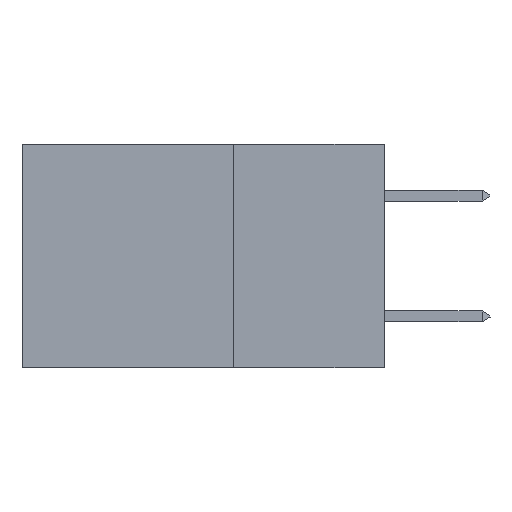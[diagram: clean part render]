
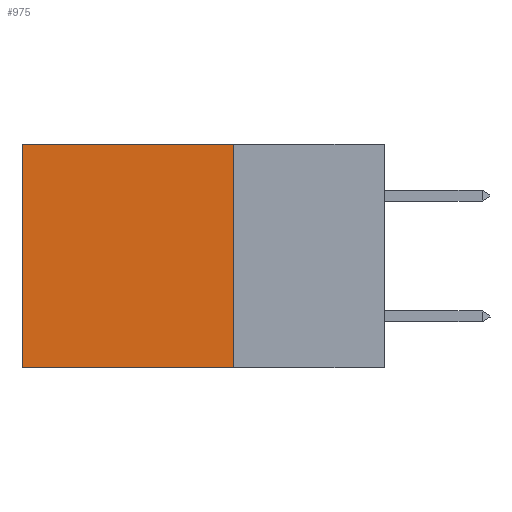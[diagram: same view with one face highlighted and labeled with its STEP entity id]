
A CAD part, left-side view. The second image highlights one B-rep face of the part: STEP entity #975.
In plain terms, the highlighted planar face has unit normal (-1, 0, 0).
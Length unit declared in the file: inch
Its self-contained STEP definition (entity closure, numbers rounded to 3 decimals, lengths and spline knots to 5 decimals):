
#78 = CARTESIAN_POINT ( 'NONE',  ( 0.2875, 0.25, 0. ) ) ;
#312 = DIRECTION ( 'NONE',  ( 0., 1., 0. ) ) ;
#412 = ORIENTED_EDGE ( 'NONE', *, *, #5667, .T. ) ;
#666 = ORIENTED_EDGE ( 'NONE', *, *, #23189, .F. ) ;
#975 = ADVANCED_FACE ( 'NONE', ( #8266 ), #23697, .F. ) ;
#1405 = CARTESIAN_POINT ( 'NONE',  ( 0.2875, 0.25, -0.37 ) ) ;
#1751 = DIRECTION ( 'NONE',  ( 0., 0., -1. ) ) ;
#2479 = CARTESIAN_POINT ( 'NONE',  ( 0.2875, 0.25, 0. ) ) ;
#2648 = LINE ( 'NONE', #6725, #13887 ) ;
#2697 = ORIENTED_EDGE ( 'NONE', *, *, #15838, .T. ) ;
#2740 = DIRECTION ( 'NONE',  ( 0., 0., -1. ) ) ;
#2899 = DIRECTION ( 'NONE',  ( 1., 0., 0. ) ) ;
#3260 = AXIS2_PLACEMENT_3D ( 'NONE', #23617, #2899, #2740 ) ;
#3999 = VECTOR ( 'NONE', #13714, 39.37008 ) ;
#4315 = LINE ( 'NONE', #2479, #3999 ) ;
#5667 = EDGE_CURVE ( 'NONE', #8730, #23796, #6262, .T. ) ;
#6262 = LINE ( 'NONE', #7137, #14560 ) ;
#6541 = CARTESIAN_POINT ( 'NONE',  ( 0.2875, 0.6, -0.37 ) ) ;
#6725 = CARTESIAN_POINT ( 'NONE',  ( 0.2875, 0.25, -0.37 ) ) ;
#7029 = CARTESIAN_POINT ( 'NONE',  ( 0.2875, 0.6, 0. ) ) ;
#7137 = CARTESIAN_POINT ( 'NONE',  ( 0.2875, 0.25, 0. ) ) ;
#8266 = FACE_OUTER_BOUND ( 'NONE', #23594, .T. ) ;
#8289 = CARTESIAN_POINT ( 'NONE',  ( 0.2875, 0.6, 0. ) ) ;
#8730 = VERTEX_POINT ( 'NONE', #78 ) ;
#9624 = EDGE_CURVE ( 'NONE', #11899, #20979, #2648, .T. ) ;
#11899 = VERTEX_POINT ( 'NONE', #1405 ) ;
#13714 = DIRECTION ( 'NONE',  ( 0., 0., -1. ) ) ;
#13887 = VECTOR ( 'NONE', #24391, 39.37008 ) ;
#14025 = LINE ( 'NONE', #7029, #23898 ) ;
#14560 = VECTOR ( 'NONE', #312, 39.37008 ) ;
#15838 = EDGE_CURVE ( 'NONE', #23796, #20979, #14025, .T. ) ;
#16441 = ORIENTED_EDGE ( 'NONE', *, *, #9624, .F. ) ;
#20979 = VERTEX_POINT ( 'NONE', #6541 ) ;
#23189 = EDGE_CURVE ( 'NONE', #8730, #11899, #4315, .T. ) ;
#23594 = EDGE_LOOP ( 'NONE', ( #2697, #16441, #666, #412 ) ) ;
#23617 = CARTESIAN_POINT ( 'NONE',  ( 0.2875, 0.25, 0. ) ) ;
#23697 = PLANE ( 'NONE',  #3260 ) ;
#23796 = VERTEX_POINT ( 'NONE', #8289 ) ;
#23898 = VECTOR ( 'NONE', #1751, 39.37008 ) ;
#24391 = DIRECTION ( 'NONE',  ( 0., 1., 0. ) ) ;
